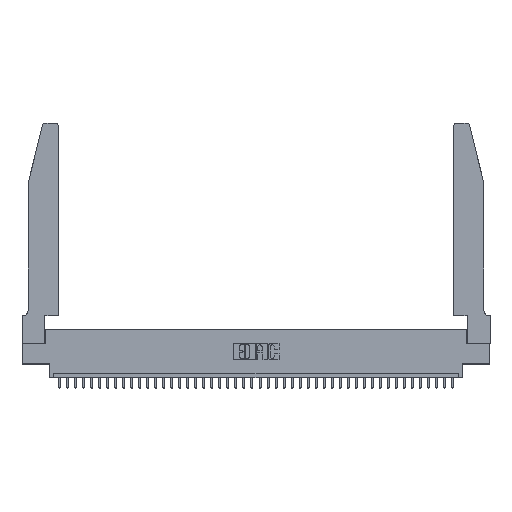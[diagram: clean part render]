
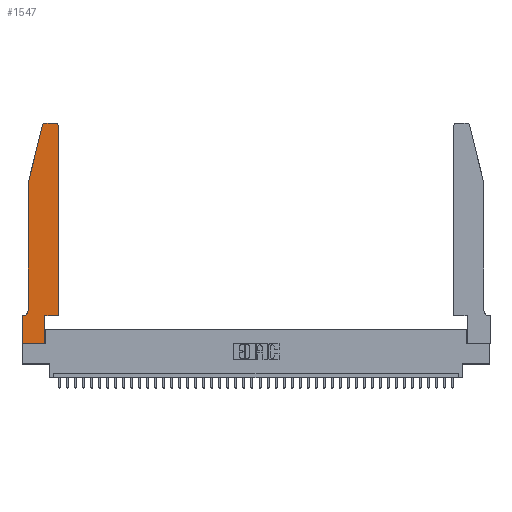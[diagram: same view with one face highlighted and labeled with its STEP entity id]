
A CAD part, top view. The second image highlights one B-rep face of the part: STEP entity #1547.
In plain terms, the highlighted planar face has unit normal (0, 0, 1).
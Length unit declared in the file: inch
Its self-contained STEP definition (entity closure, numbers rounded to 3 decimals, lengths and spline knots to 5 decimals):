
#225 = EDGE_CURVE ( 'NONE', #35037, #34738, #28191, .T. ) ;
#240 = ORIENTED_EDGE ( 'NONE', *, *, #35028, .T. ) ;
#768 = EDGE_CURVE ( 'NONE', #6358, #9298, #5157, .T. ) ;
#944 = AXIS2_PLACEMENT_3D ( 'NONE', #29334, #37751, #17581 ) ;
#1000 = ORIENTED_EDGE ( 'NONE', *, *, #41325, .T. ) ;
#1301 = CARTESIAN_POINT ( 'NONE',  ( 0.0755, 2., 0.37 ) ) ;
#1341 = CIRCLE ( 'NONE', #944, 0.03 ) ;
#1380 = CARTESIAN_POINT ( 'NONE',  ( 0., 0., 0.37 ) ) ;
#1452 = DIRECTION ( 'NONE',  ( -0.239, -0.971, 0. ) ) ;
#1547 = ADVANCED_FACE ( 'NONE', ( #18611 ), #14099, .T. ) ;
#1846 = CARTESIAN_POINT ( 'NONE',  ( 0.2865, 0.35, 0.37 ) ) ;
#2586 = CARTESIAN_POINT ( 'NONE',  ( 0.0055, 0.42, 0.37 ) ) ;
#3027 = ORIENTED_EDGE ( 'NONE', *, *, #225, .T. ) ;
#3888 = CARTESIAN_POINT ( 'NONE',  ( 0.284, 2.75, 0.37 ) ) ;
#4087 = VECTOR ( 'NONE', #17887, 39.37008 ) ;
#4247 = CARTESIAN_POINT ( 'NONE',  ( 0.4505, 0.35, 0.37 ) ) ;
#4576 = VECTOR ( 'NONE', #18723, 39.37008 ) ;
#5157 = LINE ( 'NONE', #8477, #4087 ) ;
#5562 = VERTEX_POINT ( 'NONE', #16236 ) ;
#6358 = VERTEX_POINT ( 'NONE', #33960 ) ;
#6403 = CARTESIAN_POINT ( 'NONE',  ( 0., 0., 0.37 ) ) ;
#6644 = EDGE_CURVE ( 'NONE', #37427, #20646, #30850, .T. ) ;
#7584 = ORIENTED_EDGE ( 'NONE', *, *, #36895, .T. ) ;
#7817 = VERTEX_POINT ( 'NONE', #31142 ) ;
#7867 = CARTESIAN_POINT ( 'NONE',  ( 0., 0., 0.37 ) ) ;
#7939 = CARTESIAN_POINT ( 'NONE',  ( 0.0755, 0.35, 0.37 ) ) ;
#8044 = EDGE_CURVE ( 'NONE', #12252, #11711, #22305, .T. ) ;
#8344 = ORIENTED_EDGE ( 'NONE', *, *, #25423, .T. ) ;
#8477 = CARTESIAN_POINT ( 'NONE',  ( 0.2605, 2.75, 0.37 ) ) ;
#8681 = VECTOR ( 'NONE', #14709, 39.37008 ) ;
#8692 = CARTESIAN_POINT ( 'NONE',  ( 0.0755, 2., 0.37 ) ) ;
#8740 = DIRECTION ( 'NONE',  ( 0., 0., -1. ) ) ;
#8747 = DIRECTION ( 'NONE',  ( 1., 0., 0. ) ) ;
#8769 = AXIS2_PLACEMENT_3D ( 'NONE', #2586, #8740, #18583 ) ;
#9298 = VERTEX_POINT ( 'NONE', #3888 ) ;
#10428 = CIRCLE ( 'NONE', #8769, 0.07 ) ;
#10700 = DIRECTION ( 'NONE',  ( 1., 0., 0. ) ) ;
#11047 = CARTESIAN_POINT ( 'NONE',  ( 0.4505, 0.35, 0.37 ) ) ;
#11592 = ORIENTED_EDGE ( 'NONE', *, *, #20577, .T. ) ;
#11711 = VERTEX_POINT ( 'NONE', #8692 ) ;
#11785 = DIRECTION ( 'NONE',  ( 0., 1., 0. ) ) ;
#11850 = CARTESIAN_POINT ( 'NONE',  ( 0.4505, 0.35, 0.37 ) ) ;
#12252 = VERTEX_POINT ( 'NONE', #17406 ) ;
#12513 = EDGE_CURVE ( 'NONE', #20646, #7817, #32278, .T. ) ;
#14099 = PLANE ( 'NONE',  #31133 ) ;
#14146 = ORIENTED_EDGE ( 'NONE', *, *, #8044, .T. ) ;
#14312 = VERTEX_POINT ( 'NONE', #6403 ) ;
#14709 = DIRECTION ( 'NONE',  ( -1., 0., 0. ) ) ;
#15732 = ORIENTED_EDGE ( 'NONE', *, *, #22661, .T. ) ;
#16236 = CARTESIAN_POINT ( 'NONE',  ( 0.0755, 0.42, 0.37 ) ) ;
#16945 = DIRECTION ( 'NONE',  ( 0., 0., 1. ) ) ;
#17314 = VERTEX_POINT ( 'NONE', #29247 ) ;
#17406 = CARTESIAN_POINT ( 'NONE',  ( 0.25487, 2.72718, 0.37 ) ) ;
#17581 = DIRECTION ( 'NONE',  ( 1., 0., 0. ) ) ;
#17887 = DIRECTION ( 'NONE',  ( -1., 0., 0. ) ) ;
#18355 = VECTOR ( 'NONE', #1452, 39.37008 ) ;
#18385 = VECTOR ( 'NONE', #11785, 39.37008 ) ;
#18583 = DIRECTION ( 'NONE',  ( -1., 0., 0. ) ) ;
#18611 = FACE_OUTER_BOUND ( 'NONE', #38866, .T. ) ;
#18723 = DIRECTION ( 'NONE',  ( 0., -1., 0. ) ) ;
#18975 = DIRECTION ( 'NONE',  ( 0., 1., 0. ) ) ;
#18989 = CARTESIAN_POINT ( 'NONE',  ( 0.0055, 0.35, 0.37 ) ) ;
#19106 = EDGE_CURVE ( 'NONE', #34738, #14312, #36185, .T. ) ;
#20577 = EDGE_CURVE ( 'NONE', #9298, #12252, #23040, .T. ) ;
#20646 = VERTEX_POINT ( 'NONE', #4247 ) ;
#22305 = LINE ( 'NONE', #1301, #18355 ) ;
#22661 = EDGE_CURVE ( 'NONE', #17314, #37427, #30439, .T. ) ;
#22901 = VECTOR ( 'NONE', #18975, 39.37008 ) ;
#23040 = CIRCLE ( 'NONE', #28767, 0.03 ) ;
#23430 = CARTESIAN_POINT ( 'NONE',  ( 0., 0.35, 0.37 ) ) ;
#24939 = LINE ( 'NONE', #1380, #39971 ) ;
#25423 = EDGE_CURVE ( 'NONE', #7817, #6358, #1341, .T. ) ;
#25670 = ORIENTED_EDGE ( 'NONE', *, *, #6644, .T. ) ;
#27118 = LINE ( 'NONE', #37848, #4576 ) ;
#27166 = CARTESIAN_POINT ( 'NONE',  ( 0.284, 2.72, 0.37 ) ) ;
#28191 = LINE ( 'NONE', #7939, #8681 ) ;
#28767 = AXIS2_PLACEMENT_3D ( 'NONE', #27166, #16945, #39307 ) ;
#29247 = CARTESIAN_POINT ( 'NONE',  ( 0.2865, 0., 0.37 ) ) ;
#29334 = CARTESIAN_POINT ( 'NONE',  ( 0.4205, 2.72, 0.37 ) ) ;
#30357 = VECTOR ( 'NONE', #8747, 39.37008 ) ;
#30439 = LINE ( 'NONE', #40784, #22901 ) ;
#30850 = LINE ( 'NONE', #11850, #30357 ) ;
#31133 = AXIS2_PLACEMENT_3D ( 'NONE', #23430, #36596, #10700 ) ;
#31142 = CARTESIAN_POINT ( 'NONE',  ( 0.4505, 2.72, 0.37 ) ) ;
#31681 = ORIENTED_EDGE ( 'NONE', *, *, #19106, .T. ) ;
#31744 = VECTOR ( 'NONE', #36831, 39.37008 ) ;
#32278 = LINE ( 'NONE', #11047, #18385 ) ;
#32787 = CARTESIAN_POINT ( 'NONE',  ( 0., 0.35, 0.37 ) ) ;
#33960 = CARTESIAN_POINT ( 'NONE',  ( 0.4205, 2.75, 0.37 ) ) ;
#34738 = VERTEX_POINT ( 'NONE', #32787 ) ;
#35028 = EDGE_CURVE ( 'NONE', #11711, #5562, #27118, .T. ) ;
#35037 = VERTEX_POINT ( 'NONE', #18989 ) ;
#36052 = DIRECTION ( 'NONE',  ( 1., 0., 0. ) ) ;
#36185 = LINE ( 'NONE', #7867, #31744 ) ;
#36596 = DIRECTION ( 'NONE',  ( 0., 0., 1. ) ) ;
#36831 = DIRECTION ( 'NONE',  ( 0., -1., 0. ) ) ;
#36895 = EDGE_CURVE ( 'NONE', #5562, #35037, #10428, .T. ) ;
#37427 = VERTEX_POINT ( 'NONE', #1846 ) ;
#37751 = DIRECTION ( 'NONE',  ( 0., 0., 1. ) ) ;
#37848 = CARTESIAN_POINT ( 'NONE',  ( 0.0755, 2., 0.37 ) ) ;
#38613 = ORIENTED_EDGE ( 'NONE', *, *, #768, .T. ) ;
#38866 = EDGE_LOOP ( 'NONE', ( #38613, #11592, #14146, #240, #7584, #3027, #31681, #1000, #15732, #25670, #40361, #8344 ) ) ;
#39307 = DIRECTION ( 'NONE',  ( 1., 0., 0. ) ) ;
#39971 = VECTOR ( 'NONE', #36052, 39.37008 ) ;
#40361 = ORIENTED_EDGE ( 'NONE', *, *, #12513, .T. ) ;
#40784 = CARTESIAN_POINT ( 'NONE',  ( 0.2865, 0.35, 0.37 ) ) ;
#41325 = EDGE_CURVE ( 'NONE', #14312, #17314, #24939, .T. ) ;
